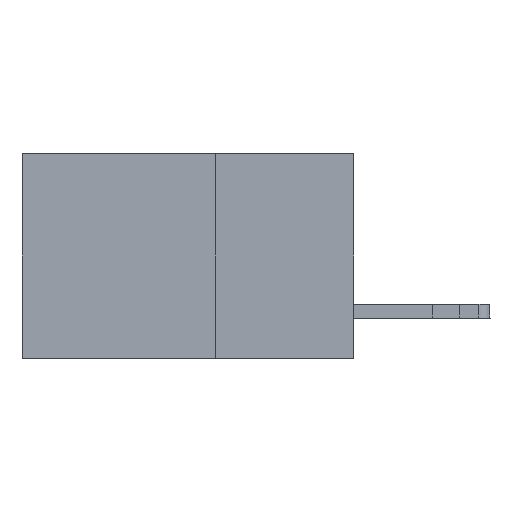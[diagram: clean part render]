
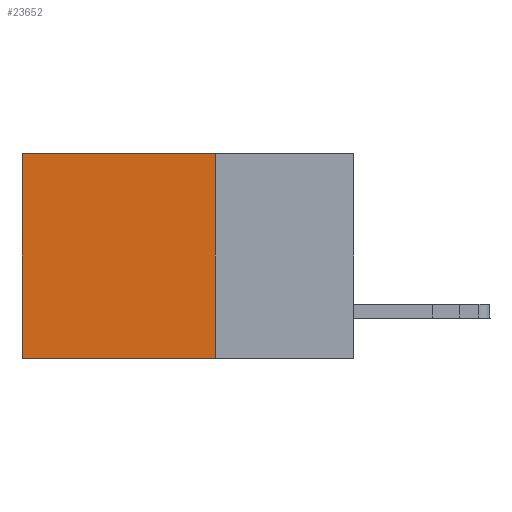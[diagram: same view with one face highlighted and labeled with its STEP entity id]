
A CAD part, left-side view. The second image highlights one B-rep face of the part: STEP entity #23652.
In plain terms, the highlighted planar face has unit normal (-1, 0, 0).
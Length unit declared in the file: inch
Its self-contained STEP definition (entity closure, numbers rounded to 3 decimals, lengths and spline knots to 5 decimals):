
#1374 = ORIENTED_EDGE ( 'NONE', *, *, #17986, .F. ) ;
#1813 = CARTESIAN_POINT ( 'NONE',  ( 0.2875, 0.25, 0. ) ) ;
#4160 = CARTESIAN_POINT ( 'NONE',  ( 0.2875, 0.25, 0. ) ) ;
#4164 = CARTESIAN_POINT ( 'NONE',  ( 0.2875, 0.6, 0. ) ) ;
#4275 = CARTESIAN_POINT ( 'NONE',  ( 0.2875, 0.6, -0.37 ) ) ;
#6165 = EDGE_CURVE ( 'NONE', #14449, #14371, #10364, .T. ) ;
#9114 = VECTOR ( 'NONE', #10450, 39.37008 ) ;
#9984 = VERTEX_POINT ( 'NONE', #4275 ) ;
#10364 = LINE ( 'NONE', #4160, #26791 ) ;
#10450 = DIRECTION ( 'NONE',  ( 0., 1., 0. ) ) ;
#11268 = PLANE ( 'NONE',  #23864 ) ;
#12050 = DIRECTION ( 'NONE',  ( 0., 0., -1. ) ) ;
#13357 = VECTOR ( 'NONE', #12050, 39.37008 ) ;
#13476 = DIRECTION ( 'NONE',  ( 0., 0., -1. ) ) ;
#13629 = DIRECTION ( 'NONE',  ( 1., 0., 0. ) ) ;
#14371 = VERTEX_POINT ( 'NONE', #4164 ) ;
#14449 = VERTEX_POINT ( 'NONE', #20892 ) ;
#14611 = VECTOR ( 'NONE', #13476, 39.37008 ) ;
#14754 = FACE_OUTER_BOUND ( 'NONE', #15536, .T. ) ;
#15536 = EDGE_LOOP ( 'NONE', ( #21988, #1374, #24128, #25729 ) ) ;
#16425 = EDGE_CURVE ( 'NONE', #14449, #27851, #25051, .T. ) ;
#16683 = CARTESIAN_POINT ( 'NONE',  ( 0.2875, 0.25, -0.37 ) ) ;
#17986 = EDGE_CURVE ( 'NONE', #27851, #9984, #21545, .T. ) ;
#20892 = CARTESIAN_POINT ( 'NONE',  ( 0.2875, 0.25, 0. ) ) ;
#21545 = LINE ( 'NONE', #22098, #9114 ) ;
#21558 = LINE ( 'NONE', #27469, #14611 ) ;
#21988 = ORIENTED_EDGE ( 'NONE', *, *, #26423, .T. ) ;
#22098 = CARTESIAN_POINT ( 'NONE',  ( 0.2875, 0.25, -0.37 ) ) ;
#23652 = ADVANCED_FACE ( 'NONE', ( #14754 ), #11268, .F. ) ;
#23864 = AXIS2_PLACEMENT_3D ( 'NONE', #1813, #13629, #29935 ) ;
#24128 = ORIENTED_EDGE ( 'NONE', *, *, #16425, .F. ) ;
#25051 = LINE ( 'NONE', #26060, #13357 ) ;
#25729 = ORIENTED_EDGE ( 'NONE', *, *, #6165, .T. ) ;
#26060 = CARTESIAN_POINT ( 'NONE',  ( 0.2875, 0.25, 0. ) ) ;
#26423 = EDGE_CURVE ( 'NONE', #14371, #9984, #21558, .T. ) ;
#26791 = VECTOR ( 'NONE', #27617, 39.37008 ) ;
#27469 = CARTESIAN_POINT ( 'NONE',  ( 0.2875, 0.6, 0. ) ) ;
#27617 = DIRECTION ( 'NONE',  ( 0., 1., 0. ) ) ;
#27851 = VERTEX_POINT ( 'NONE', #16683 ) ;
#29935 = DIRECTION ( 'NONE',  ( 0., 0., -1. ) ) ;
